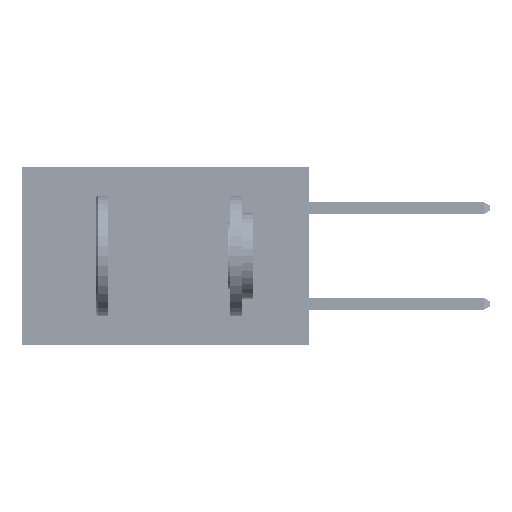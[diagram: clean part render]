
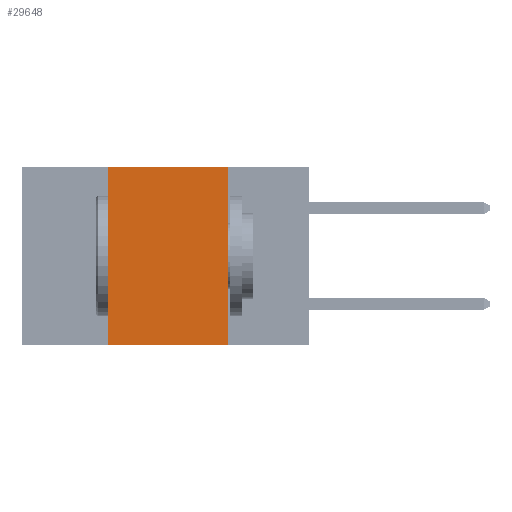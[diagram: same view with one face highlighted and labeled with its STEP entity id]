
A CAD part, left-side view. The second image highlights one B-rep face of the part: STEP entity #29648.
In plain terms, the highlighted planar face has unit normal (-1, 0, 0).
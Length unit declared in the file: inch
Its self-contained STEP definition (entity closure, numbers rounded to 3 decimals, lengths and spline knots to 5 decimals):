
#1007 = EDGE_CURVE ( 'NONE', #47878, #4277, #10177, .T. ) ;
#1461 = DIRECTION ( 'NONE',  ( 1., 0., 0. ) ) ;
#1941 = DIRECTION ( 'NONE',  ( 0., -1., 0. ) ) ;
#4277 = VERTEX_POINT ( 'NONE', #10900 ) ;
#5305 = CARTESIAN_POINT ( 'NONE',  ( 0., 0.17, 0. ) ) ;
#5545 = CARTESIAN_POINT ( 'NONE',  ( 0., 0.6, 0. ) ) ;
#5733 = PLANE ( 'NONE',  #39879 ) ;
#7386 = EDGE_CURVE ( 'NONE', #27534, #39642, #15838, .T. ) ;
#8420 = CARTESIAN_POINT ( 'NONE',  ( 0., 0.42, 0. ) ) ;
#8723 = FACE_OUTER_BOUND ( 'NONE', #32862, .T. ) ;
#8767 = CARTESIAN_POINT ( 'NONE',  ( 0., 0.42, -0.37 ) ) ;
#8929 = VECTOR ( 'NONE', #42696, 39.37008 ) ;
#9600 = EDGE_CURVE ( 'NONE', #27534, #4277, #14096, .T. ) ;
#10177 = LINE ( 'NONE', #29746, #8929 ) ;
#10900 = CARTESIAN_POINT ( 'NONE',  ( 0., 0.17, -0.37 ) ) ;
#14096 = LINE ( 'NONE', #25567, #17115 ) ;
#14670 = ORIENTED_EDGE ( 'NONE', *, *, #17450, .F. ) ;
#15838 = LINE ( 'NONE', #36214, #27469 ) ;
#16539 = ORIENTED_EDGE ( 'NONE', *, *, #7386, .F. ) ;
#17115 = VECTOR ( 'NONE', #1941, 39.37008 ) ;
#17450 = EDGE_CURVE ( 'NONE', #39642, #47878, #43486, .T. ) ;
#25567 = CARTESIAN_POINT ( 'NONE',  ( 0., 0.6, -0.37 ) ) ;
#27469 = VECTOR ( 'NONE', #48504, 39.37008 ) ;
#27534 = VERTEX_POINT ( 'NONE', #8767 ) ;
#29444 = ORIENTED_EDGE ( 'NONE', *, *, #9600, .T. ) ;
#29648 = ADVANCED_FACE ( 'NONE', ( #8723 ), #5733, .F. ) ;
#29746 = CARTESIAN_POINT ( 'NONE',  ( 0., 0.17, 0. ) ) ;
#32862 = EDGE_LOOP ( 'NONE', ( #42425, #14670, #16539, #29444 ) ) ;
#33153 = DIRECTION ( 'NONE',  ( 0., 0., -1. ) ) ;
#33157 = VECTOR ( 'NONE', #34605, 39.37008 ) ;
#34605 = DIRECTION ( 'NONE',  ( 0., -1., 0. ) ) ;
#36214 = CARTESIAN_POINT ( 'NONE',  ( 0., 0.42, 0. ) ) ;
#39642 = VERTEX_POINT ( 'NONE', #8420 ) ;
#39879 = AXIS2_PLACEMENT_3D ( 'NONE', #5545, #1461, #33153 ) ;
#42425 = ORIENTED_EDGE ( 'NONE', *, *, #1007, .F. ) ;
#42598 = CARTESIAN_POINT ( 'NONE',  ( 0., 0.6, 0. ) ) ;
#42696 = DIRECTION ( 'NONE',  ( 0., 0., -1. ) ) ;
#43486 = LINE ( 'NONE', #42598, #33157 ) ;
#47878 = VERTEX_POINT ( 'NONE', #5305 ) ;
#48504 = DIRECTION ( 'NONE',  ( 0., 0., 1. ) ) ;
